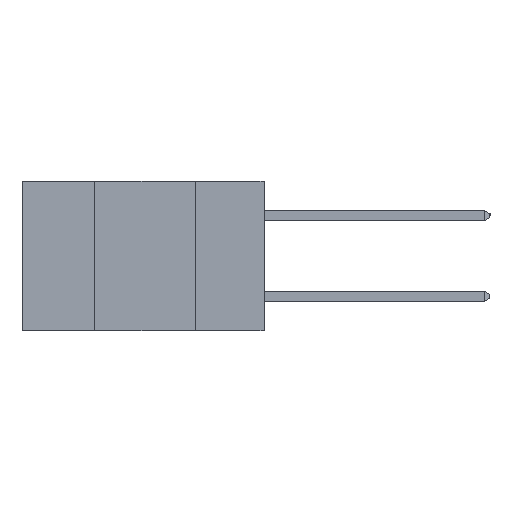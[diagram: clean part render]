
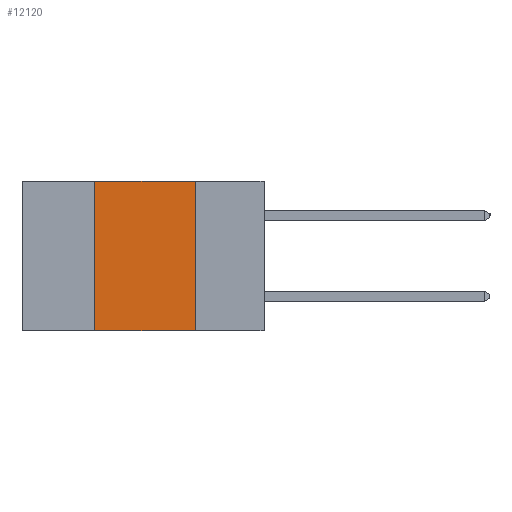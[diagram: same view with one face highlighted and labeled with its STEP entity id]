
A CAD part, left-side view. The second image highlights one B-rep face of the part: STEP entity #12120.
In plain terms, the highlighted planar face has unit normal (-1, 0, 0).
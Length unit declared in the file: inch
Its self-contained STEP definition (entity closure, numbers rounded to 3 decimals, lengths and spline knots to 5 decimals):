
#355 = CARTESIAN_POINT ( 'NONE',  ( 0., 0.17, 0. ) ) ;
#629 = LINE ( 'NONE', #11128, #10636 ) ;
#862 = PLANE ( 'NONE',  #3425 ) ;
#1984 = ORIENTED_EDGE ( 'NONE', *, *, #6109, .T. ) ;
#2886 = DIRECTION ( 'NONE',  ( 0., -1., 0. ) ) ;
#3425 = AXIS2_PLACEMENT_3D ( 'NONE', #15974, #15593, #18671 ) ;
#3762 = EDGE_CURVE ( 'NONE', #12007, #8016, #8419, .T. ) ;
#4446 = LINE ( 'NONE', #14721, #7978 ) ;
#6109 = EDGE_CURVE ( 'NONE', #10297, #10683, #4446, .T. ) ;
#6565 = EDGE_LOOP ( 'NONE', ( #7745, #19123, #6643, #1984 ) ) ;
#6643 = ORIENTED_EDGE ( 'NONE', *, *, #13686, .F. ) ;
#6962 = DIRECTION ( 'NONE',  ( 0., -1., 0. ) ) ;
#7745 = ORIENTED_EDGE ( 'NONE', *, *, #15598, .F. ) ;
#7852 = CARTESIAN_POINT ( 'NONE',  ( 0., 0.42, 0. ) ) ;
#7978 = VECTOR ( 'NONE', #2886, 39.37008 ) ;
#8016 = VERTEX_POINT ( 'NONE', #355 ) ;
#8334 = FACE_OUTER_BOUND ( 'NONE', #6565, .T. ) ;
#8419 = LINE ( 'NONE', #13240, #13533 ) ;
#9888 = LINE ( 'NONE', #15881, #17365 ) ;
#10297 = VERTEX_POINT ( 'NONE', #16458 ) ;
#10636 = VECTOR ( 'NONE', #10845, 39.37008 ) ;
#10683 = VERTEX_POINT ( 'NONE', #10779 ) ;
#10779 = CARTESIAN_POINT ( 'NONE',  ( 0., 0.17, -0.37 ) ) ;
#10845 = DIRECTION ( 'NONE',  ( 0., 0., -1. ) ) ;
#11128 = CARTESIAN_POINT ( 'NONE',  ( 0., 0.17, -0.37 ) ) ;
#12007 = VERTEX_POINT ( 'NONE', #7852 ) ;
#12120 = ADVANCED_FACE ( 'NONE', ( #8334 ), #862, .F. ) ;
#13240 = CARTESIAN_POINT ( 'NONE',  ( 0., 0.6, 0. ) ) ;
#13533 = VECTOR ( 'NONE', #6962, 39.37008 ) ;
#13686 = EDGE_CURVE ( 'NONE', #10297, #12007, #9888, .T. ) ;
#14721 = CARTESIAN_POINT ( 'NONE',  ( 0., 0.6, -0.37 ) ) ;
#15593 = DIRECTION ( 'NONE',  ( 1., 0., 0. ) ) ;
#15598 = EDGE_CURVE ( 'NONE', #8016, #10683, #629, .T. ) ;
#15881 = CARTESIAN_POINT ( 'NONE',  ( 0., 0.42, -0.37 ) ) ;
#15974 = CARTESIAN_POINT ( 'NONE',  ( 0., 0.6, 0. ) ) ;
#16458 = CARTESIAN_POINT ( 'NONE',  ( 0., 0.42, -0.37 ) ) ;
#17365 = VECTOR ( 'NONE', #17511, 39.37008 ) ;
#17511 = DIRECTION ( 'NONE',  ( 0., 0., 1. ) ) ;
#18671 = DIRECTION ( 'NONE',  ( 0., 0., -1. ) ) ;
#19123 = ORIENTED_EDGE ( 'NONE', *, *, #3762, .F. ) ;
